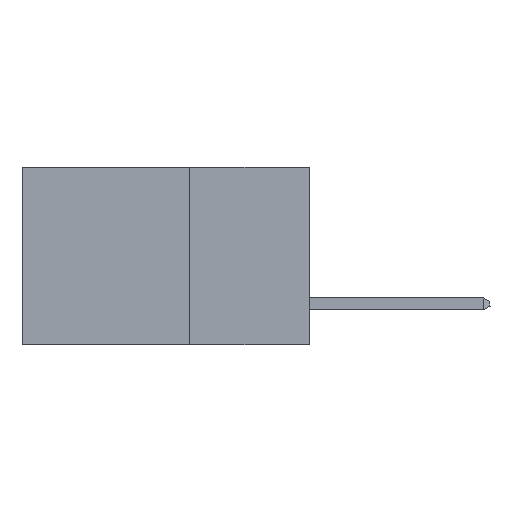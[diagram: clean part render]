
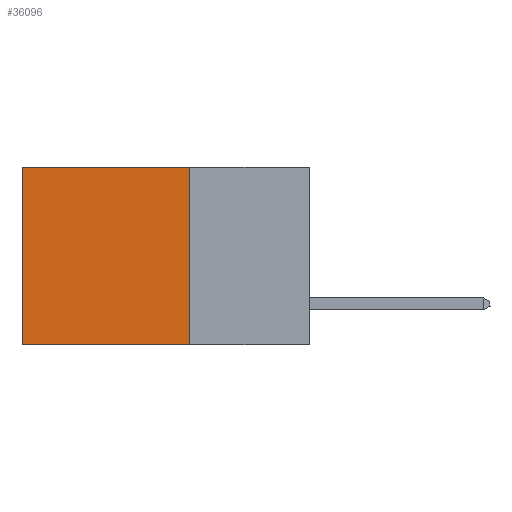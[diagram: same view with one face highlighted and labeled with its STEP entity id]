
A CAD part, left-side view. The second image highlights one B-rep face of the part: STEP entity #36096.
In plain terms, the highlighted planar face has unit normal (-1, 0, 0).
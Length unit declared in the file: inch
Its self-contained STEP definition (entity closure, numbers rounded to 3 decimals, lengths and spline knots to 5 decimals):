
#1068 = AXIS2_PLACEMENT_3D ( 'NONE', #25179, #10897, #4552 ) ;
#2473 = CARTESIAN_POINT ( 'NONE',  ( 0.2875, 0.25, 0. ) ) ;
#3689 = VERTEX_POINT ( 'NONE', #17161 ) ;
#4113 = ORIENTED_EDGE ( 'NONE', *, *, #42929, .T. ) ;
#4552 = DIRECTION ( 'NONE',  ( 0., 0., -1. ) ) ;
#5381 = EDGE_LOOP ( 'NONE', ( #4113, #37917, #7358, #23238 ) ) ;
#5398 = CARTESIAN_POINT ( 'NONE',  ( 0.2875, 0.25, -0.37 ) ) ;
#7358 = ORIENTED_EDGE ( 'NONE', *, *, #35828, .F. ) ;
#9295 = VECTOR ( 'NONE', #22671, 39.37008 ) ;
#10897 = DIRECTION ( 'NONE',  ( 1., 0., 0. ) ) ;
#11077 = VECTOR ( 'NONE', #33612, 39.37008 ) ;
#15949 = LINE ( 'NONE', #2473, #41727 ) ;
#17161 = CARTESIAN_POINT ( 'NONE',  ( 0.2875, 0.6, -0.37 ) ) ;
#19282 = CARTESIAN_POINT ( 'NONE',  ( 0.2875, 0.25, 0. ) ) ;
#21730 = PLANE ( 'NONE',  #1068 ) ;
#21760 = VECTOR ( 'NONE', #27557, 39.37008 ) ;
#22671 = DIRECTION ( 'NONE',  ( 0., 0., -1. ) ) ;
#23238 = ORIENTED_EDGE ( 'NONE', *, *, #40957, .T. ) ;
#25179 = CARTESIAN_POINT ( 'NONE',  ( 0.2875, 0.25, 0. ) ) ;
#27277 = VERTEX_POINT ( 'NONE', #5398 ) ;
#27557 = DIRECTION ( 'NONE',  ( 0., 1., 0. ) ) ;
#27625 = CARTESIAN_POINT ( 'NONE',  ( 0.2875, 0.6, 0. ) ) ;
#30624 = VERTEX_POINT ( 'NONE', #32370 ) ;
#31008 = LINE ( 'NONE', #19282, #11077 ) ;
#31280 = EDGE_CURVE ( 'NONE', #27277, #3689, #35259, .T. ) ;
#32370 = CARTESIAN_POINT ( 'NONE',  ( 0.2875, 0.25, 0. ) ) ;
#33612 = DIRECTION ( 'NONE',  ( 0., 1., 0. ) ) ;
#35004 = CARTESIAN_POINT ( 'NONE',  ( 0.2875, 0.25, -0.37 ) ) ;
#35259 = LINE ( 'NONE', #35004, #21760 ) ;
#35828 = EDGE_CURVE ( 'NONE', #30624, #27277, #15949, .T. ) ;
#35838 = VERTEX_POINT ( 'NONE', #27625 ) ;
#36096 = ADVANCED_FACE ( 'NONE', ( #44487 ), #21730, .F. ) ;
#37917 = ORIENTED_EDGE ( 'NONE', *, *, #31280, .F. ) ;
#40957 = EDGE_CURVE ( 'NONE', #30624, #35838, #31008, .T. ) ;
#41727 = VECTOR ( 'NONE', #43888, 39.37008 ) ;
#42929 = EDGE_CURVE ( 'NONE', #35838, #3689, #43740, .T. ) ;
#43247 = CARTESIAN_POINT ( 'NONE',  ( 0.2875, 0.6, 0. ) ) ;
#43740 = LINE ( 'NONE', #43247, #9295 ) ;
#43888 = DIRECTION ( 'NONE',  ( 0., 0., -1. ) ) ;
#44487 = FACE_OUTER_BOUND ( 'NONE', #5381, .T. ) ;
